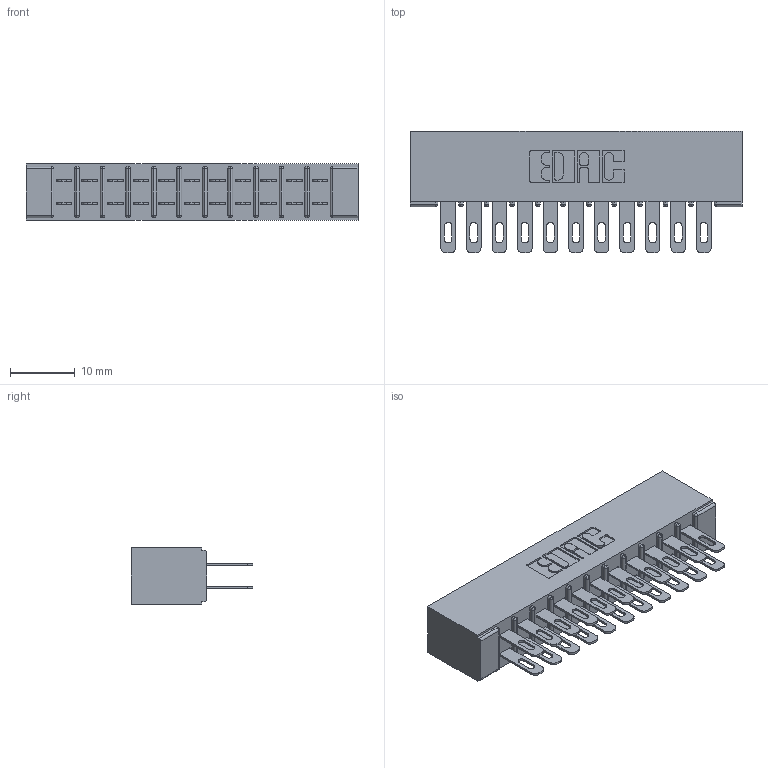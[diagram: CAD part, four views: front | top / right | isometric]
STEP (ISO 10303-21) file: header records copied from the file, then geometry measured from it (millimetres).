
FILE_DESCRIPTION (( 'STEP AP203' ), '1' );
FILE_NAME ('355-022-500-501.STEP', '2019-09-11T03:50:35', ( '' ), ( '' ), 'SwSTEP 2.0', 'SolidWorks 2016', '' );
FILE_SCHEMA (( 'CONFIG_CONTROL_DESIGN' ));
Length unit declared in the file: inch
Products named in the file (3): 305 Part_No Mounting; 305-290-001_500; 355-022-500-501
Assembly tree (23 placements, depth 2):
  355-022-500-501
    305 Part_No Mounting
    305-290-001_500  x22
Bounding box: 51.46 x 18.85 x 8.71 mm (x, y, z)
Volume: 3343.5 mm3; surface area: 6980.2 mm2
Topology: 23 solids, 23 shells, 1208 faces, 3449 edges, 2238 vertices
Faces by surface type: plane 680, cylinder 484, sphere 44
Entity records: 15428 total; most frequent: CARTESIAN_POINT 2551, ORIENTED_EDGE 2526, DIRECTION 2493, EDGE_CURVE 1263, VECTOR 989, LINE 989, VERTEX_POINT 810, AXIS2_PLACEMENT_3D 752
